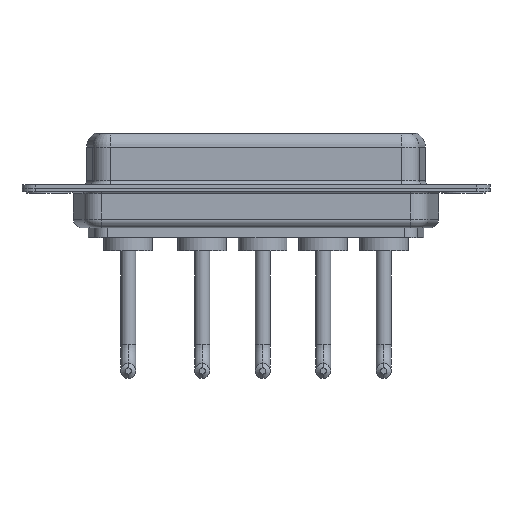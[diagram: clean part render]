
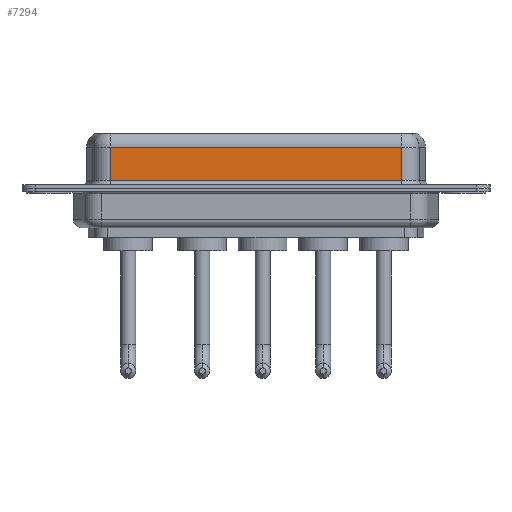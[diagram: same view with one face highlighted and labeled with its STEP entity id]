
A CAD part, front view. The second image highlights one B-rep face of the part: STEP entity #7294.
In plain terms, the highlighted planar face has unit normal (0, -1, 0).
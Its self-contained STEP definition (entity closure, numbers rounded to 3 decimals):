
#165 = DIRECTION ( 'NONE',  ( 0., 1., 0. ) ) ;
#186 = LINE ( 'NONE', #6998, #5742 ) ;
#1064 = ORIENTED_EDGE ( 'NONE', *, *, #7030, .T. ) ;
#1434 = EDGE_CURVE ( 'NONE', #8678, #6327, #4461, .T. ) ;
#2005 = LINE ( 'NONE', #8924, #4665 ) ;
#2589 = CARTESIAN_POINT ( 'NONE',  ( 40.037, -3.95, 6.4 ) ) ;
#2662 = EDGE_LOOP ( 'NONE', ( #6187, #7883, #1064, #5357 ) ) ;
#2685 = VECTOR ( 'NONE', #10395, 1000. ) ;
#3716 = DIRECTION ( 'NONE',  ( 0., 0., -1. ) ) ;
#4461 = LINE ( 'NONE', #8891, #2685 ) ;
#4665 = VECTOR ( 'NONE', #3716, 1000. ) ;
#4991 = CARTESIAN_POINT ( 'NONE',  ( 40.037, -3.95, 4.65 ) ) ;
#5357 = ORIENTED_EDGE ( 'NONE', *, *, #8470, .T. ) ;
#5731 = VECTOR ( 'NONE', #10864, 1000. ) ;
#5742 = VECTOR ( 'NONE', #6484, 1000. ) ;
#5970 = DIRECTION ( 'NONE',  ( 0., 0., 1. ) ) ;
#6021 = FACE_OUTER_BOUND ( 'NONE', #2662, .T. ) ;
#6187 = ORIENTED_EDGE ( 'NONE', *, *, #1434, .F. ) ;
#6327 = VERTEX_POINT ( 'NONE', #9554 ) ;
#6484 = DIRECTION ( 'NONE',  ( 1., 0., 0. ) ) ;
#6545 = VERTEX_POINT ( 'NONE', #10546 ) ;
#6705 = LINE ( 'NONE', #7485, #5731 ) ;
#6998 = CARTESIAN_POINT ( 'NONE',  ( 40.037, -3.95, 0.9 ) ) ;
#7030 = EDGE_CURVE ( 'NONE', #10381, #6545, #2005, .T. ) ;
#7294 = ADVANCED_FACE ( 'NONE', ( #6021 ), #10200, .F. ) ;
#7485 = CARTESIAN_POINT ( 'NONE',  ( 40.037, -3.95, 4.65 ) ) ;
#7883 = ORIENTED_EDGE ( 'NONE', *, *, #8056, .T. ) ;
#8056 = EDGE_CURVE ( 'NONE', #8678, #10381, #6705, .T. ) ;
#8470 = EDGE_CURVE ( 'NONE', #6545, #6327, #186, .T. ) ;
#8678 = VERTEX_POINT ( 'NONE', #4991 ) ;
#8891 = CARTESIAN_POINT ( 'NONE',  ( 40.037, -3.95, 6.4 ) ) ;
#8917 = AXIS2_PLACEMENT_3D ( 'NONE', #2589, #165, #5970 ) ;
#8924 = CARTESIAN_POINT ( 'NONE',  ( 7.013, -3.95, 6.4 ) ) ;
#9554 = CARTESIAN_POINT ( 'NONE',  ( 40.037, -3.95, 0.9 ) ) ;
#10029 = CARTESIAN_POINT ( 'NONE',  ( 7.013, -3.95, 4.65 ) ) ;
#10200 = PLANE ( 'NONE',  #8917 ) ;
#10381 = VERTEX_POINT ( 'NONE', #10029 ) ;
#10395 = DIRECTION ( 'NONE',  ( 0., 0., -1. ) ) ;
#10546 = CARTESIAN_POINT ( 'NONE',  ( 7.013, -3.95, 0.9 ) ) ;
#10864 = DIRECTION ( 'NONE',  ( -1., 0., 0. ) ) ;
